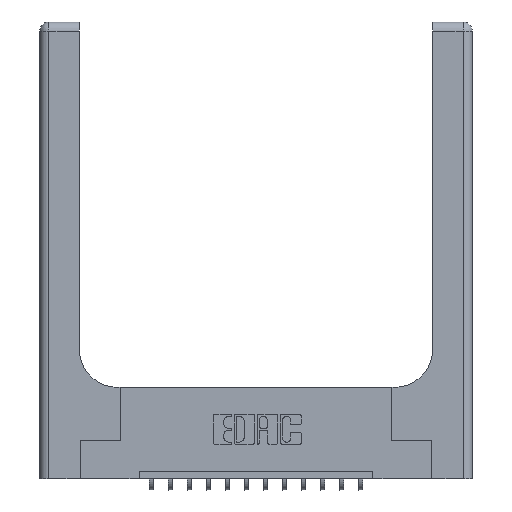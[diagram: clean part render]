
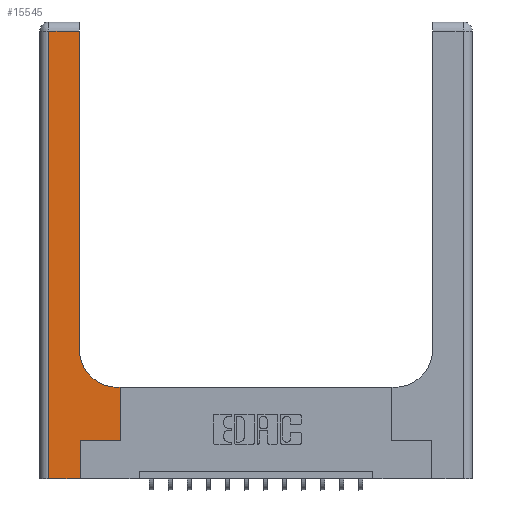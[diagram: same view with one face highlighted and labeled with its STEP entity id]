
A CAD part, top view. The second image highlights one B-rep face of the part: STEP entity #15545.
In plain terms, the highlighted planar face has unit normal (0, 0, 1).
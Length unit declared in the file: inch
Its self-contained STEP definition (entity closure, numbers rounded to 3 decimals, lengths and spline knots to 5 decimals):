
#657 = ORIENTED_EDGE ( 'NONE', *, *, #11691, .T. ) ;
#1176 = CARTESIAN_POINT ( 'NONE',  ( 0.528, 0.25, 0.37 ) ) ;
#1317 = DIRECTION ( 'NONE',  ( 1., 0., 0. ) ) ;
#1339 = CARTESIAN_POINT ( 'NONE',  ( 0.265, 0.25, 0.37 ) ) ;
#1420 = LINE ( 'NONE', #1339, #13425 ) ;
#1564 = PLANE ( 'NONE',  #7259 ) ;
#1608 = AXIS2_PLACEMENT_3D ( 'NONE', #8648, #13922, #12614 ) ;
#1725 = ORIENTED_EDGE ( 'NONE', *, *, #7478, .T. ) ;
#1930 = CARTESIAN_POINT ( 'NONE',  ( 0.51, 0.6, 0.37 ) ) ;
#2529 = DIRECTION ( 'NONE',  ( 0., 0., -1. ) ) ;
#2600 = ORIENTED_EDGE ( 'NONE', *, *, #12036, .T. ) ;
#2777 = DIRECTION ( 'NONE',  ( -1., 0., 0. ) ) ;
#3368 = DIRECTION ( 'NONE',  ( -1., 0., 0. ) ) ;
#3418 = ORIENTED_EDGE ( 'NONE', *, *, #16644, .T. ) ;
#3473 = DIRECTION ( 'NONE',  ( 0., 1., 0. ) ) ;
#4202 = CARTESIAN_POINT ( 'NONE',  ( 0.06, 3., 0.37 ) ) ;
#4336 = CARTESIAN_POINT ( 'NONE',  ( 0.26, 0.85, 0.37 ) ) ;
#4679 = ORIENTED_EDGE ( 'NONE', *, *, #5550, .T. ) ;
#4836 = EDGE_CURVE ( 'NONE', #6024, #9355, #11062, .T. ) ;
#5052 = CARTESIAN_POINT ( 'NONE',  ( 0., 0., 0.37 ) ) ;
#5055 = LINE ( 'NONE', #15828, #5956 ) ;
#5286 = LINE ( 'NONE', #9204, #16443 ) ;
#5550 = EDGE_CURVE ( 'NONE', #8133, #6441, #5286, .T. ) ;
#5585 = VERTEX_POINT ( 'NONE', #7912 ) ;
#5792 = VERTEX_POINT ( 'NONE', #8674 ) ;
#5956 = VECTOR ( 'NONE', #15913, 39.37008 ) ;
#6024 = VERTEX_POINT ( 'NONE', #1176 ) ;
#6441 = VERTEX_POINT ( 'NONE', #9833 ) ;
#6516 = ORIENTED_EDGE ( 'NONE', *, *, #6748, .T. ) ;
#6748 = EDGE_CURVE ( 'NONE', #14771, #5792, #15739, .T. ) ;
#6869 = FACE_OUTER_BOUND ( 'NONE', #16603, .T. ) ;
#7259 = AXIS2_PLACEMENT_3D ( 'NONE', #7935, #2529, #2777 ) ;
#7478 = EDGE_CURVE ( 'NONE', #5792, #15008, #16103, .T. ) ;
#7713 = VERTEX_POINT ( 'NONE', #1930 ) ;
#7781 = DIRECTION ( 'NONE',  ( 1., 0., 0. ) ) ;
#7912 = CARTESIAN_POINT ( 'NONE',  ( 0.06, 2.94, 0.37 ) ) ;
#7935 = CARTESIAN_POINT ( 'NONE',  ( 0., 3., 0.37 ) ) ;
#8133 = VERTEX_POINT ( 'NONE', #4336 ) ;
#8648 = CARTESIAN_POINT ( 'NONE',  ( 0.51, 0.85, 0.37 ) ) ;
#8674 = CARTESIAN_POINT ( 'NONE',  ( 0.265, 0., 0.37 ) ) ;
#8720 = VECTOR ( 'NONE', #17064, 39.37008 ) ;
#9204 = CARTESIAN_POINT ( 'NONE',  ( 0.26, 3., 0.37 ) ) ;
#9274 = ORIENTED_EDGE ( 'NONE', *, *, #13765, .T. ) ;
#9355 = VERTEX_POINT ( 'NONE', #11809 ) ;
#9518 = DIRECTION ( 'NONE',  ( 0., -1., 0. ) ) ;
#9618 = VECTOR ( 'NONE', #9518, 39.37008 ) ;
#9833 = CARTESIAN_POINT ( 'NONE',  ( 0.26, 2.94, 0.37 ) ) ;
#9981 = LINE ( 'NONE', #15282, #11549 ) ;
#10202 = CIRCLE ( 'NONE', #1608, 0.25 ) ;
#10860 = VECTOR ( 'NONE', #3473, 39.37008 ) ;
#11062 = LINE ( 'NONE', #13500, #10860 ) ;
#11549 = VECTOR ( 'NONE', #3368, 39.37008 ) ;
#11691 = EDGE_CURVE ( 'NONE', #5585, #14771, #16120, .T. ) ;
#11809 = CARTESIAN_POINT ( 'NONE',  ( 0.528, 0.6, 0.37 ) ) ;
#12036 = EDGE_CURVE ( 'NONE', #6441, #5585, #9981, .T. ) ;
#12614 = DIRECTION ( 'NONE',  ( 1., 0., 0. ) ) ;
#12839 = VECTOR ( 'NONE', #1317, 39.37008 ) ;
#13425 = VECTOR ( 'NONE', #7781, 39.37008 ) ;
#13483 = CARTESIAN_POINT ( 'NONE',  ( 0.265, 0., 0.37 ) ) ;
#13500 = CARTESIAN_POINT ( 'NONE',  ( 0.528, 0.25, 0.37 ) ) ;
#13531 = ORIENTED_EDGE ( 'NONE', *, *, #17040, .T. ) ;
#13765 = EDGE_CURVE ( 'NONE', #7713, #8133, #10202, .T. ) ;
#13922 = DIRECTION ( 'NONE',  ( 0., 0., -1. ) ) ;
#14493 = DIRECTION ( 'NONE',  ( 0., 1., 0. ) ) ;
#14771 = VERTEX_POINT ( 'NONE', #16036 ) ;
#14991 = ORIENTED_EDGE ( 'NONE', *, *, #4836, .T. ) ;
#15008 = VERTEX_POINT ( 'NONE', #16798 ) ;
#15282 = CARTESIAN_POINT ( 'NONE',  ( 0., 2.94, 0.37 ) ) ;
#15545 = ADVANCED_FACE ( 'NONE', ( #6869 ), #1564, .F. ) ;
#15739 = LINE ( 'NONE', #5052, #12839 ) ;
#15828 = CARTESIAN_POINT ( 'NONE',  ( 0.26, 0.6, 0.37 ) ) ;
#15913 = DIRECTION ( 'NONE',  ( -1., 0., 0. ) ) ;
#16036 = CARTESIAN_POINT ( 'NONE',  ( 0.06, 0., 0.37 ) ) ;
#16103 = LINE ( 'NONE', #13483, #8720 ) ;
#16120 = LINE ( 'NONE', #4202, #9618 ) ;
#16443 = VECTOR ( 'NONE', #14493, 39.37008 ) ;
#16603 = EDGE_LOOP ( 'NONE', ( #4679, #2600, #657, #6516, #1725, #3418, #14991, #13531, #9274 ) ) ;
#16644 = EDGE_CURVE ( 'NONE', #15008, #6024, #1420, .T. ) ;
#16798 = CARTESIAN_POINT ( 'NONE',  ( 0.265, 0.25, 0.37 ) ) ;
#17040 = EDGE_CURVE ( 'NONE', #9355, #7713, #5055, .T. ) ;
#17064 = DIRECTION ( 'NONE',  ( 0., 1., 0. ) ) ;
